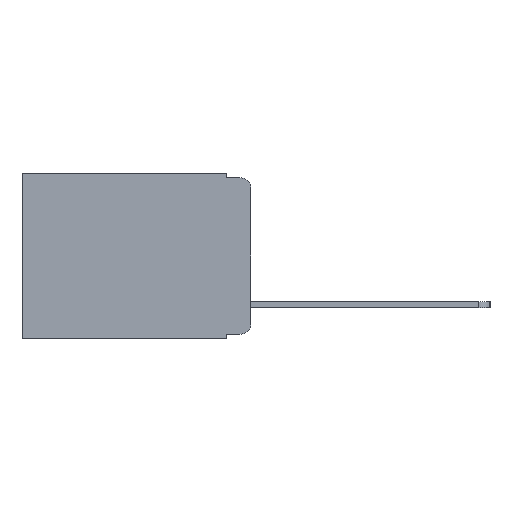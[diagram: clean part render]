
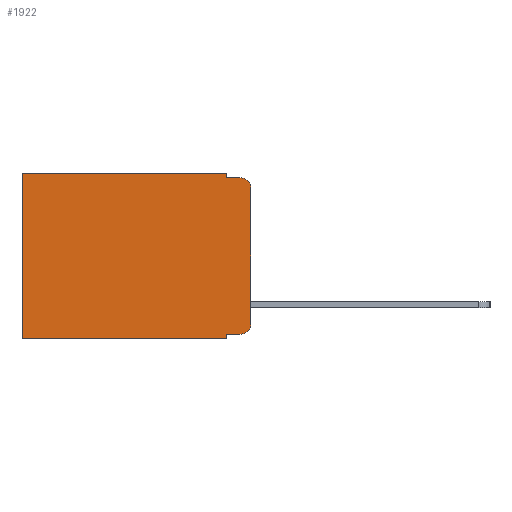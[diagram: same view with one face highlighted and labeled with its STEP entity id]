
A CAD part, left-side view. The second image highlights one B-rep face of the part: STEP entity #1922.
In plain terms, the highlighted planar face has unit normal (-1, 0, 0).
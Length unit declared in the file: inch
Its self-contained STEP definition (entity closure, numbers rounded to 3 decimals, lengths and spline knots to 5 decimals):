
#287 = DIRECTION ( 'NONE',  ( 0., 1., 0. ) ) ;
#291 = VERTEX_POINT ( 'NONE', #12710 ) ;
#492 = ORIENTED_EDGE ( 'NONE', *, *, #2875, .T. ) ;
#686 = DIRECTION ( 'NONE',  ( 0., 0., -1. ) ) ;
#708 = FACE_OUTER_BOUND ( 'NONE', #10741, .T. ) ;
#853 = LINE ( 'NONE', #1378, #4442 ) ;
#997 = DIRECTION ( 'NONE',  ( 0., 0., -1. ) ) ;
#1344 = VERTEX_POINT ( 'NONE', #1479 ) ;
#1378 = CARTESIAN_POINT ( 'NONE',  ( 0.298, 0.051, -0.333 ) ) ;
#1479 = CARTESIAN_POINT ( 'NONE',  ( 0.298, 0.051, 0. ) ) ;
#1922 = ADVANCED_FACE ( 'NONE', ( #708 ), #10775, .F. ) ;
#2449 = CARTESIAN_POINT ( 'NONE',  ( 0.298, 0., -0.343 ) ) ;
#2541 = CARTESIAN_POINT ( 'NONE',  ( 0.298, 0.473, 0. ) ) ;
#2590 = AXIS2_PLACEMENT_3D ( 'NONE', #8692, #8744, #8781 ) ;
#2592 = CARTESIAN_POINT ( 'NONE',  ( 0.298, 0.473, 0. ) ) ;
#2872 = CIRCLE ( 'NONE', #2590, 0.02 ) ;
#2875 = EDGE_CURVE ( 'NONE', #15235, #15133, #2872, .T. ) ;
#3067 = VECTOR ( 'NONE', #16594, 39.37008 ) ;
#3866 = EDGE_CURVE ( 'NONE', #5357, #15235, #853, .T. ) ;
#3883 = ORIENTED_EDGE ( 'NONE', *, *, #14559, .F. ) ;
#4337 = CIRCLE ( 'NONE', #4745, 0.02 ) ;
#4426 = AXIS2_PLACEMENT_3D ( 'NONE', #7119, #14802, #14962 ) ;
#4442 = VECTOR ( 'NONE', #6993, 39.37008 ) ;
#4543 = ORIENTED_EDGE ( 'NONE', *, *, #11201, .T. ) ;
#4610 = ORIENTED_EDGE ( 'NONE', *, *, #9465, .F. ) ;
#4745 = AXIS2_PLACEMENT_3D ( 'NONE', #5468, #14606, #6836 ) ;
#5243 = ORIENTED_EDGE ( 'NONE', *, *, #7681, .F. ) ;
#5357 = VERTEX_POINT ( 'NONE', #14229 ) ;
#5431 = LINE ( 'NONE', #2592, #11721 ) ;
#5468 = CARTESIAN_POINT ( 'NONE',  ( 0.298, 0.02, -0.03 ) ) ;
#5797 = EDGE_CURVE ( 'NONE', #5357, #7351, #16655, .T. ) ;
#5969 = VERTEX_POINT ( 'NONE', #8940 ) ;
#6439 = LINE ( 'NONE', #15462, #3067 ) ;
#6725 = EDGE_CURVE ( 'NONE', #14177, #5969, #5431, .T. ) ;
#6836 = DIRECTION ( 'NONE',  ( 0., 0., -1. ) ) ;
#6993 = DIRECTION ( 'NONE',  ( 0., -1., 0. ) ) ;
#7014 = CARTESIAN_POINT ( 'NONE',  ( 0.298, 0.051, -0.343 ) ) ;
#7119 = CARTESIAN_POINT ( 'NONE',  ( 0.298, 0., 0. ) ) ;
#7351 = VERTEX_POINT ( 'NONE', #7014 ) ;
#7384 = ORIENTED_EDGE ( 'NONE', *, *, #10253, .T. ) ;
#7411 = LINE ( 'NONE', #8650, #10547 ) ;
#7681 = EDGE_CURVE ( 'NONE', #1344, #12272, #6439, .T. ) ;
#8198 = CARTESIAN_POINT ( 'NONE',  ( 0.298, 0.051, -0.01 ) ) ;
#8650 = CARTESIAN_POINT ( 'NONE',  ( 0.298, 0., 0. ) ) ;
#8692 = CARTESIAN_POINT ( 'NONE',  ( 0.298, 0.02, -0.313 ) ) ;
#8744 = DIRECTION ( 'NONE',  ( -1., 0., 0. ) ) ;
#8781 = DIRECTION ( 'NONE',  ( 0., 0., -1. ) ) ;
#8816 = VECTOR ( 'NONE', #14564, 39.37008 ) ;
#8940 = CARTESIAN_POINT ( 'NONE',  ( 0.298, 0.473, -0.343 ) ) ;
#9253 = LINE ( 'NONE', #2449, #8816 ) ;
#9465 = EDGE_CURVE ( 'NONE', #12272, #14895, #10626, .T. ) ;
#9996 = DIRECTION ( 'NONE',  ( 0., 0., -1. ) ) ;
#10253 = EDGE_CURVE ( 'NONE', #1344, #14177, #10594, .T. ) ;
#10389 = ORIENTED_EDGE ( 'NONE', *, *, #6725, .T. ) ;
#10547 = VECTOR ( 'NONE', #9996, 39.37008 ) ;
#10594 = LINE ( 'NONE', #16474, #13594 ) ;
#10626 = LINE ( 'NONE', #8198, #16753 ) ;
#10741 = EDGE_LOOP ( 'NONE', ( #3883, #4543, #4610, #5243, #7384, #10389, #14402, #14505, #14763, #492 ) ) ;
#10775 = PLANE ( 'NONE',  #4426 ) ;
#11201 = EDGE_CURVE ( 'NONE', #291, #14895, #4337, .T. ) ;
#11325 = CARTESIAN_POINT ( 'NONE',  ( 0.298, 0.051, -0.01 ) ) ;
#11721 = VECTOR ( 'NONE', #997, 39.37008 ) ;
#12272 = VERTEX_POINT ( 'NONE', #11325 ) ;
#12710 = CARTESIAN_POINT ( 'NONE',  ( 0.298, 0., -0.03 ) ) ;
#13139 = VECTOR ( 'NONE', #686, 39.37008 ) ;
#13594 = VECTOR ( 'NONE', #287, 39.37008 ) ;
#14041 = CARTESIAN_POINT ( 'NONE',  ( 0.298, 0.02, -0.333 ) ) ;
#14177 = VERTEX_POINT ( 'NONE', #2541 ) ;
#14229 = CARTESIAN_POINT ( 'NONE',  ( 0.298, 0.051, -0.333 ) ) ;
#14402 = ORIENTED_EDGE ( 'NONE', *, *, #17346, .F. ) ;
#14417 = CARTESIAN_POINT ( 'NONE',  ( 0.298, 0.02, -0.01 ) ) ;
#14505 = ORIENTED_EDGE ( 'NONE', *, *, #5797, .F. ) ;
#14559 = EDGE_CURVE ( 'NONE', #291, #15133, #7411, .T. ) ;
#14564 = DIRECTION ( 'NONE',  ( 0., 1., 0. ) ) ;
#14606 = DIRECTION ( 'NONE',  ( -1., 0., 0. ) ) ;
#14763 = ORIENTED_EDGE ( 'NONE', *, *, #3866, .T. ) ;
#14802 = DIRECTION ( 'NONE',  ( 1., 0., 0. ) ) ;
#14895 = VERTEX_POINT ( 'NONE', #14417 ) ;
#14962 = DIRECTION ( 'NONE',  ( 0., 0., -1. ) ) ;
#15133 = VERTEX_POINT ( 'NONE', #17041 ) ;
#15235 = VERTEX_POINT ( 'NONE', #14041 ) ;
#15462 = CARTESIAN_POINT ( 'NONE',  ( 0.298, 0.051, 0. ) ) ;
#16474 = CARTESIAN_POINT ( 'NONE',  ( 0.298, 0., 0. ) ) ;
#16594 = DIRECTION ( 'NONE',  ( 0., 0., -1. ) ) ;
#16655 = LINE ( 'NONE', #16868, #13139 ) ;
#16753 = VECTOR ( 'NONE', #16898, 39.37008 ) ;
#16868 = CARTESIAN_POINT ( 'NONE',  ( 0.298, 0.051, 0. ) ) ;
#16898 = DIRECTION ( 'NONE',  ( 0., -1., 0. ) ) ;
#17041 = CARTESIAN_POINT ( 'NONE',  ( 0.298, 0., -0.313 ) ) ;
#17346 = EDGE_CURVE ( 'NONE', #7351, #5969, #9253, .T. ) ;
